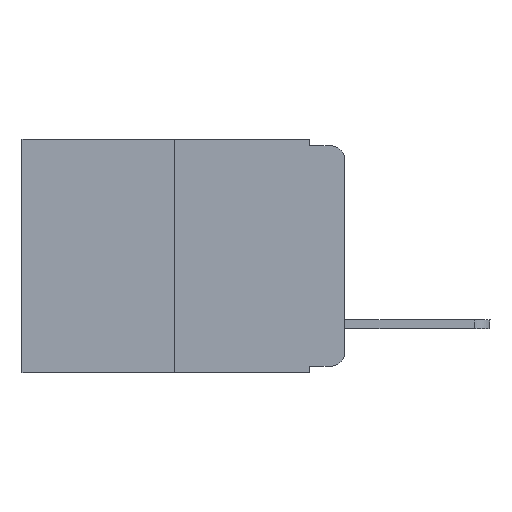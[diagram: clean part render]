
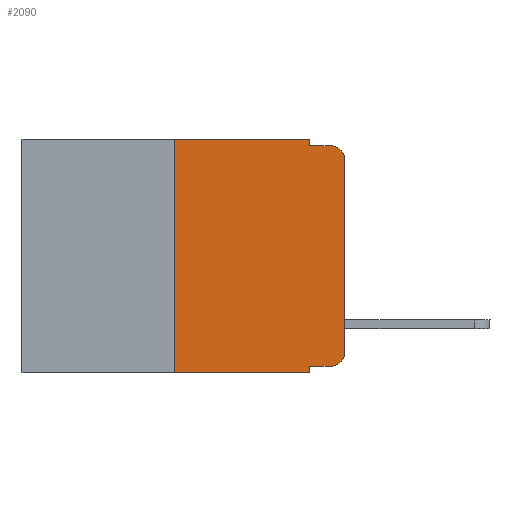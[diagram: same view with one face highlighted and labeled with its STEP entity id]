
A CAD part, left-side view. The second image highlights one B-rep face of the part: STEP entity #2090.
In plain terms, the highlighted planar face has unit normal (-1, 0, 0).
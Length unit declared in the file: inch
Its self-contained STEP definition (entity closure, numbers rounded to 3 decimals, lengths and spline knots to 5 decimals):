
#93 = CARTESIAN_POINT ( 'NONE',  ( 0., 0.02, -0.333 ) ) ;
#316 = CARTESIAN_POINT ( 'NONE',  ( 0., 0.051, 0. ) ) ;
#438 = VERTEX_POINT ( 'NONE', #4093 ) ;
#730 = LINE ( 'NONE', #12533, #13042 ) ;
#768 = EDGE_CURVE ( 'NONE', #13693, #438, #790, .T. ) ;
#790 = LINE ( 'NONE', #3287, #12908 ) ;
#1122 = EDGE_LOOP ( 'NONE', ( #9635, #7834, #1741, #13985, #6505, #4626, #5282, #10526, #14147, #7310 ) ) ;
#1741 = ORIENTED_EDGE ( 'NONE', *, *, #10095, .F. ) ;
#2090 = ADVANCED_FACE ( 'NONE', ( #10767 ), #8273, .F. ) ;
#2198 = EDGE_CURVE ( 'NONE', #2282, #13448, #730, .T. ) ;
#2282 = VERTEX_POINT ( 'NONE', #4910 ) ;
#2780 = VECTOR ( 'NONE', #4501, 39.37008 ) ;
#3040 = DIRECTION ( 'NONE',  ( 0., 0., 1. ) ) ;
#3093 = DIRECTION ( 'NONE',  ( 0., -1., 0. ) ) ;
#3287 = CARTESIAN_POINT ( 'NONE',  ( 0., 0., 0. ) ) ;
#3569 = LINE ( 'NONE', #8859, #14399 ) ;
#3827 = EDGE_CURVE ( 'NONE', #16194, #14541, #14380, .T. ) ;
#4093 = CARTESIAN_POINT ( 'NONE',  ( 0., 0., -0.03 ) ) ;
#4501 = DIRECTION ( 'NONE',  ( 0., 0., -1. ) ) ;
#4626 = ORIENTED_EDGE ( 'NONE', *, *, #12355, .F. ) ;
#4654 = VERTEX_POINT ( 'NONE', #93 ) ;
#4752 = DIRECTION ( 'NONE',  ( 0., -1., 0. ) ) ;
#4910 = CARTESIAN_POINT ( 'NONE',  ( 0., 0.25, -0.343 ) ) ;
#4912 = DIRECTION ( 'NONE',  ( -1., 0., 0. ) ) ;
#5065 = CARTESIAN_POINT ( 'NONE',  ( 0., 0.473, 0. ) ) ;
#5282 = ORIENTED_EDGE ( 'NONE', *, *, #2198, .T. ) ;
#6155 = DIRECTION ( 'NONE',  ( 0., -1., 0. ) ) ;
#6505 = ORIENTED_EDGE ( 'NONE', *, *, #7133, .F. ) ;
#7133 = EDGE_CURVE ( 'NONE', #15491, #16194, #12688, .T. ) ;
#7310 = ORIENTED_EDGE ( 'NONE', *, *, #8347, .T. ) ;
#7359 = AXIS2_PLACEMENT_3D ( 'NONE', #15228, #4912, #8937 ) ;
#7360 = DIRECTION ( 'NONE',  ( 0., 0., 1. ) ) ;
#7834 = ORIENTED_EDGE ( 'NONE', *, *, #9967, .T. ) ;
#7838 = EDGE_CURVE ( 'NONE', #10695, #4654, #15848, .T. ) ;
#7928 = CARTESIAN_POINT ( 'NONE',  ( 0., 0.051, 0. ) ) ;
#8048 = EDGE_CURVE ( 'NONE', #10695, #13448, #13379, .T. ) ;
#8273 = PLANE ( 'NONE',  #13373 ) ;
#8347 = EDGE_CURVE ( 'NONE', #4654, #13693, #8418, .T. ) ;
#8418 = CIRCLE ( 'NONE', #7359, 0.02 ) ;
#8836 = LINE ( 'NONE', #10341, #9182 ) ;
#8859 = CARTESIAN_POINT ( 'NONE',  ( 0., 0.25, 0. ) ) ;
#8937 = DIRECTION ( 'NONE',  ( 0., 0., -1. ) ) ;
#8949 = CARTESIAN_POINT ( 'NONE',  ( 0., 0., -0.313 ) ) ;
#9182 = VECTOR ( 'NONE', #6155, 39.37008 ) ;
#9346 = VECTOR ( 'NONE', #13192, 39.37008 ) ;
#9361 = DIRECTION ( 'NONE',  ( 1., 0., 0. ) ) ;
#9471 = CARTESIAN_POINT ( 'NONE',  ( 0., 0.051, -0.333 ) ) ;
#9635 = ORIENTED_EDGE ( 'NONE', *, *, #768, .T. ) ;
#9762 = DIRECTION ( 'NONE',  ( -1., 0., 0. ) ) ;
#9967 = EDGE_CURVE ( 'NONE', #438, #12056, #12913, .T. ) ;
#10095 = EDGE_CURVE ( 'NONE', #14541, #12056, #8836, .T. ) ;
#10341 = CARTESIAN_POINT ( 'NONE',  ( 0., 0.051, -0.01 ) ) ;
#10526 = ORIENTED_EDGE ( 'NONE', *, *, #8048, .F. ) ;
#10695 = VERTEX_POINT ( 'NONE', #11654 ) ;
#10767 = FACE_OUTER_BOUND ( 'NONE', #1122, .T. ) ;
#10855 = DIRECTION ( 'NONE',  ( 0., 0., -1. ) ) ;
#11654 = CARTESIAN_POINT ( 'NONE',  ( 0., 0.051, -0.333 ) ) ;
#11719 = CARTESIAN_POINT ( 'NONE',  ( 0., 0.051, -0.343 ) ) ;
#12056 = VERTEX_POINT ( 'NONE', #15575 ) ;
#12355 = EDGE_CURVE ( 'NONE', #2282, #15491, #3569, .T. ) ;
#12519 = CARTESIAN_POINT ( 'NONE',  ( 0., 0.02, -0.03 ) ) ;
#12533 = CARTESIAN_POINT ( 'NONE',  ( 0., 0.473, -0.343 ) ) ;
#12688 = LINE ( 'NONE', #5065, #16467 ) ;
#12850 = DIRECTION ( 'NONE',  ( 0., -1., 0. ) ) ;
#12908 = VECTOR ( 'NONE', #3040, 39.37008 ) ;
#12913 = CIRCLE ( 'NONE', #15069, 0.02 ) ;
#13042 = VECTOR ( 'NONE', #4752, 39.37008 ) ;
#13192 = DIRECTION ( 'NONE',  ( 0., 0., -1. ) ) ;
#13373 = AXIS2_PLACEMENT_3D ( 'NONE', #15898, #9361, #10855 ) ;
#13379 = LINE ( 'NONE', #14649, #2780 ) ;
#13448 = VERTEX_POINT ( 'NONE', #11719 ) ;
#13693 = VERTEX_POINT ( 'NONE', #8949 ) ;
#13694 = DIRECTION ( 'NONE',  ( 0., 0., -1. ) ) ;
#13985 = ORIENTED_EDGE ( 'NONE', *, *, #3827, .F. ) ;
#14084 = CARTESIAN_POINT ( 'NONE',  ( 0., 0.051, -0.01 ) ) ;
#14147 = ORIENTED_EDGE ( 'NONE', *, *, #7838, .T. ) ;
#14380 = LINE ( 'NONE', #7928, #9346 ) ;
#14399 = VECTOR ( 'NONE', #7360, 39.37008 ) ;
#14541 = VERTEX_POINT ( 'NONE', #14084 ) ;
#14649 = CARTESIAN_POINT ( 'NONE',  ( 0., 0.051, 0. ) ) ;
#14837 = VECTOR ( 'NONE', #3093, 39.37008 ) ;
#15069 = AXIS2_PLACEMENT_3D ( 'NONE', #12519, #9762, #13694 ) ;
#15228 = CARTESIAN_POINT ( 'NONE',  ( 0., 0.02, -0.313 ) ) ;
#15388 = CARTESIAN_POINT ( 'NONE',  ( 0., 0.25, 0. ) ) ;
#15491 = VERTEX_POINT ( 'NONE', #15388 ) ;
#15575 = CARTESIAN_POINT ( 'NONE',  ( 0., 0.02, -0.01 ) ) ;
#15848 = LINE ( 'NONE', #9471, #14837 ) ;
#15898 = CARTESIAN_POINT ( 'NONE',  ( 0., 0.473, 0. ) ) ;
#16194 = VERTEX_POINT ( 'NONE', #316 ) ;
#16467 = VECTOR ( 'NONE', #12850, 39.37008 ) ;
